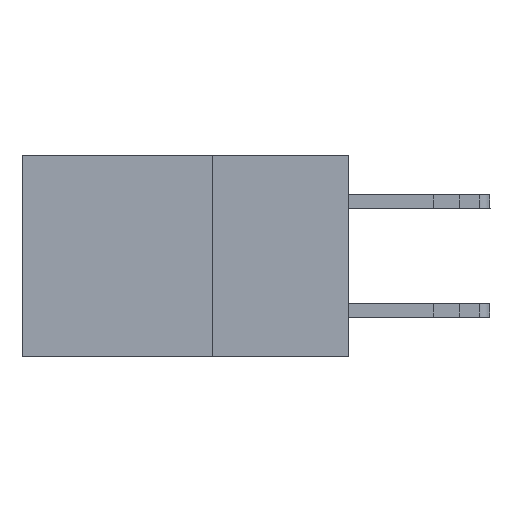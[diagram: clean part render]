
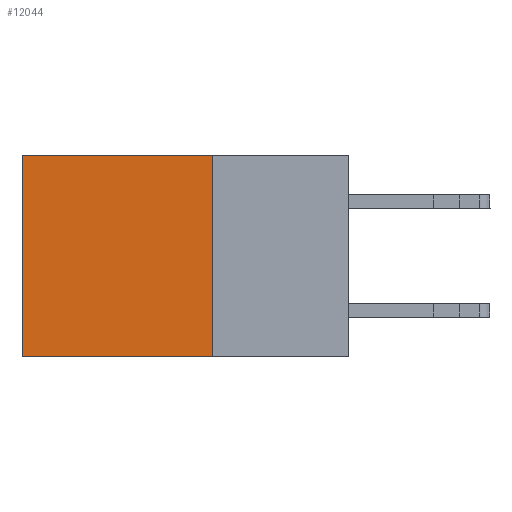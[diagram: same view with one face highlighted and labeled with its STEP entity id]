
A CAD part, left-side view. The second image highlights one B-rep face of the part: STEP entity #12044.
In plain terms, the highlighted planar face has unit normal (-1, 0, 0).
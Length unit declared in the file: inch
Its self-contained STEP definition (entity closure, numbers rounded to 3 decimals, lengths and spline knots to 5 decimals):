
#109 = LINE ( 'NONE', #3853, #11586 ) ;
#126 = ORIENTED_EDGE ( 'NONE', *, *, #6655, .F. ) ;
#1023 = DIRECTION ( 'NONE',  ( 0., 0., -1. ) ) ;
#1556 = ORIENTED_EDGE ( 'NONE', *, *, #6426, .T. ) ;
#1576 = ORIENTED_EDGE ( 'NONE', *, *, #5857, .T. ) ;
#2459 = LINE ( 'NONE', #8155, #9857 ) ;
#2924 = DIRECTION ( 'NONE',  ( 1., 0., 0. ) ) ;
#3185 = CARTESIAN_POINT ( 'NONE',  ( 0.2615, 0.25, -0.37 ) ) ;
#3238 = VERTEX_POINT ( 'NONE', #10951 ) ;
#3664 = VERTEX_POINT ( 'NONE', #9898 ) ;
#3853 = CARTESIAN_POINT ( 'NONE',  ( 0.2615, 0.25, -0.37 ) ) ;
#3886 = CARTESIAN_POINT ( 'NONE',  ( 0.2615, 0.25, 0. ) ) ;
#3945 = DIRECTION ( 'NONE',  ( 0., 1., 0. ) ) ;
#3986 = CARTESIAN_POINT ( 'NONE',  ( 0.2615, 0.25, 0. ) ) ;
#4327 = EDGE_CURVE ( 'NONE', #9945, #3238, #109, .T. ) ;
#4694 = FACE_OUTER_BOUND ( 'NONE', #8126, .T. ) ;
#4891 = ORIENTED_EDGE ( 'NONE', *, *, #4327, .F. ) ;
#4985 = LINE ( 'NONE', #3886, #8499 ) ;
#5631 = LINE ( 'NONE', #9350, #7535 ) ;
#5857 = EDGE_CURVE ( 'NONE', #11013, #3664, #4985, .T. ) ;
#6133 = DIRECTION ( 'NONE',  ( 0., 0., -1. ) ) ;
#6426 = EDGE_CURVE ( 'NONE', #3664, #3238, #2459, .T. ) ;
#6655 = EDGE_CURVE ( 'NONE', #11013, #9945, #5631, .T. ) ;
#7119 = AXIS2_PLACEMENT_3D ( 'NONE', #10444, #2924, #1023 ) ;
#7535 = VECTOR ( 'NONE', #10328, 39.37008 ) ;
#8126 = EDGE_LOOP ( 'NONE', ( #1556, #4891, #126, #1576 ) ) ;
#8155 = CARTESIAN_POINT ( 'NONE',  ( 0.2615, 0.6, -0.37 ) ) ;
#8499 = VECTOR ( 'NONE', #3945, 39.37008 ) ;
#8574 = DIRECTION ( 'NONE',  ( 0., 1., 0. ) ) ;
#9350 = CARTESIAN_POINT ( 'NONE',  ( 0.2615, 0.25, -0.37 ) ) ;
#9857 = VECTOR ( 'NONE', #6133, 39.37008 ) ;
#9898 = CARTESIAN_POINT ( 'NONE',  ( 0.2615, 0.6, 0. ) ) ;
#9945 = VERTEX_POINT ( 'NONE', #3185 ) ;
#10328 = DIRECTION ( 'NONE',  ( 0., 0., -1. ) ) ;
#10444 = CARTESIAN_POINT ( 'NONE',  ( 0.2615, 0.25, -0.37 ) ) ;
#10951 = CARTESIAN_POINT ( 'NONE',  ( 0.2615, 0.6, -0.37 ) ) ;
#11013 = VERTEX_POINT ( 'NONE', #3986 ) ;
#11309 = PLANE ( 'NONE',  #7119 ) ;
#11586 = VECTOR ( 'NONE', #8574, 39.37008 ) ;
#12044 = ADVANCED_FACE ( 'NONE', ( #4694 ), #11309, .F. ) ;
